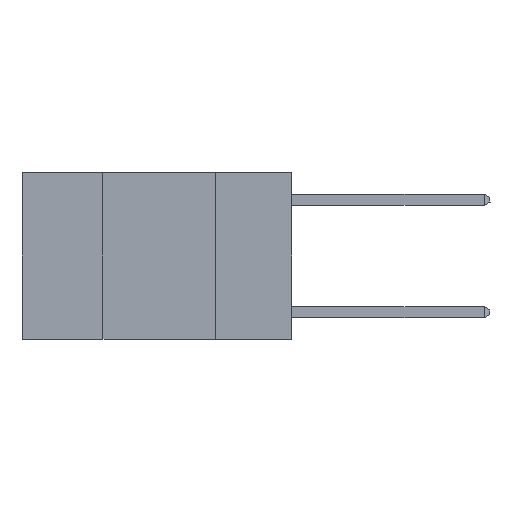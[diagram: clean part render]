
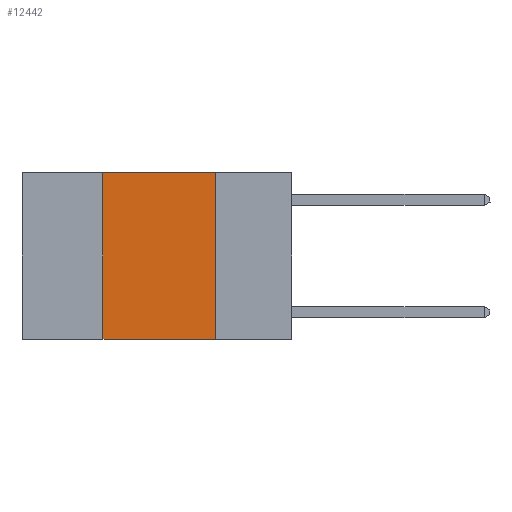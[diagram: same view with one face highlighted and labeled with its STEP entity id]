
A CAD part, left-side view. The second image highlights one B-rep face of the part: STEP entity #12442.
In plain terms, the highlighted planar face has unit normal (-1, 0, 0).
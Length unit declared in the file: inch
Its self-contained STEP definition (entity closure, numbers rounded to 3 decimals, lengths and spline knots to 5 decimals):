
#438 = VERTEX_POINT ( 'NONE', #2097 ) ;
#555 = DIRECTION ( 'NONE',  ( 0., 0., 1. ) ) ;
#964 = DIRECTION ( 'NONE',  ( 0., -1., 0. ) ) ;
#2097 = CARTESIAN_POINT ( 'NONE',  ( 0., 0.42, 0. ) ) ;
#2217 = CARTESIAN_POINT ( 'NONE',  ( 0., 0.17, 0. ) ) ;
#2758 = AXIS2_PLACEMENT_3D ( 'NONE', #10439, #24866, #12518 ) ;
#4387 = LINE ( 'NONE', #11291, #25689 ) ;
#4629 = CARTESIAN_POINT ( 'NONE',  ( 0., 0.42, 0. ) ) ;
#4746 = CARTESIAN_POINT ( 'NONE',  ( 0., 0.42, -0.37 ) ) ;
#4791 = EDGE_CURVE ( 'NONE', #23862, #17319, #22426, .T. ) ;
#4844 = EDGE_CURVE ( 'NONE', #26197, #17319, #25958, .T. ) ;
#5535 = CARTESIAN_POINT ( 'NONE',  ( 0., 0.17, -0.37 ) ) ;
#5980 = VECTOR ( 'NONE', #14398, 39.37008 ) ;
#6257 = ORIENTED_EDGE ( 'NONE', *, *, #23291, .F. ) ;
#6289 = PLANE ( 'NONE',  #2758 ) ;
#6419 = LINE ( 'NONE', #4629, #21590 ) ;
#8421 = DIRECTION ( 'NONE',  ( 0., 0., -1. ) ) ;
#10439 = CARTESIAN_POINT ( 'NONE',  ( 0., 0.6, 0. ) ) ;
#11291 = CARTESIAN_POINT ( 'NONE',  ( 0., 0.6, 0. ) ) ;
#12442 = ADVANCED_FACE ( 'NONE', ( #21507 ), #6289, .F. ) ;
#12518 = DIRECTION ( 'NONE',  ( 0., 0., -1. ) ) ;
#14398 = DIRECTION ( 'NONE',  ( 0., -1., 0. ) ) ;
#16184 = CARTESIAN_POINT ( 'NONE',  ( 0., 0.17, 0. ) ) ;
#16575 = ORIENTED_EDGE ( 'NONE', *, *, #4844, .F. ) ;
#17319 = VERTEX_POINT ( 'NONE', #5535 ) ;
#18767 = EDGE_LOOP ( 'NONE', ( #16575, #6257, #19704, #25022 ) ) ;
#19135 = EDGE_CURVE ( 'NONE', #23862, #438, #6419, .T. ) ;
#19704 = ORIENTED_EDGE ( 'NONE', *, *, #19135, .F. ) ;
#20487 = VECTOR ( 'NONE', #8421, 39.37008 ) ;
#20631 = CARTESIAN_POINT ( 'NONE',  ( 0., 0.6, -0.37 ) ) ;
#21507 = FACE_OUTER_BOUND ( 'NONE', #18767, .T. ) ;
#21590 = VECTOR ( 'NONE', #555, 39.37008 ) ;
#22426 = LINE ( 'NONE', #20631, #5980 ) ;
#23291 = EDGE_CURVE ( 'NONE', #438, #26197, #4387, .T. ) ;
#23862 = VERTEX_POINT ( 'NONE', #4746 ) ;
#24866 = DIRECTION ( 'NONE',  ( 1., 0., 0. ) ) ;
#25022 = ORIENTED_EDGE ( 'NONE', *, *, #4791, .T. ) ;
#25689 = VECTOR ( 'NONE', #964, 39.37008 ) ;
#25958 = LINE ( 'NONE', #2217, #20487 ) ;
#26197 = VERTEX_POINT ( 'NONE', #16184 ) ;
